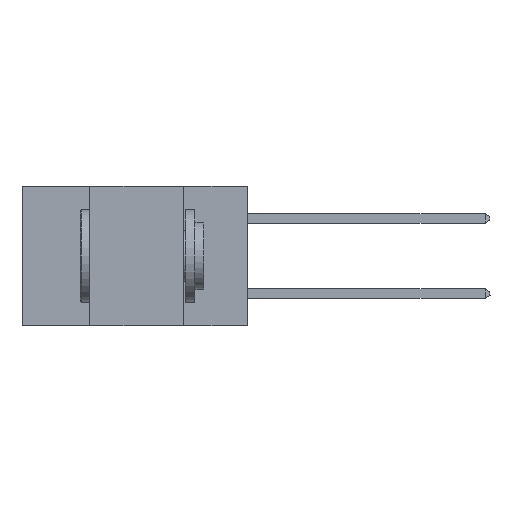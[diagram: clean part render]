
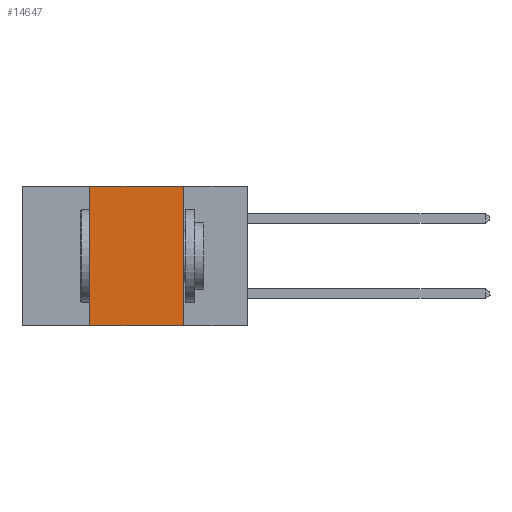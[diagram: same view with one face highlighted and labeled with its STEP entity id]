
A CAD part, left-side view. The second image highlights one B-rep face of the part: STEP entity #14647.
In plain terms, the highlighted planar face has unit normal (-1, 0, 0).
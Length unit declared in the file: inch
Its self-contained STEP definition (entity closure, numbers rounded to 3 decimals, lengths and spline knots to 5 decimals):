
#562 = PLANE ( 'NONE',  #14080 ) ;
#1736 = CARTESIAN_POINT ( 'NONE',  ( 0., 0.17, 0. ) ) ;
#3290 = VECTOR ( 'NONE', #17499, 39.37008 ) ;
#3989 = ORIENTED_EDGE ( 'NONE', *, *, #22649, .F. ) ;
#4442 = VERTEX_POINT ( 'NONE', #15856 ) ;
#6640 = CARTESIAN_POINT ( 'NONE',  ( 0., 0.6, 0. ) ) ;
#7183 = VECTOR ( 'NONE', #24436, 39.37008 ) ;
#7204 = ORIENTED_EDGE ( 'NONE', *, *, #22754, .T. ) ;
#7404 = LINE ( 'NONE', #11483, #8375 ) ;
#7886 = ORIENTED_EDGE ( 'NONE', *, *, #10504, .F. ) ;
#8375 = VECTOR ( 'NONE', #13555, 39.37008 ) ;
#9929 = VERTEX_POINT ( 'NONE', #11337 ) ;
#10027 = LINE ( 'NONE', #10076, #7183 ) ;
#10076 = CARTESIAN_POINT ( 'NONE',  ( 0., 0.42, 0. ) ) ;
#10504 = EDGE_CURVE ( 'NONE', #4442, #9929, #18807, .T. ) ;
#11337 = CARTESIAN_POINT ( 'NONE',  ( 0., 0.17, -0.37 ) ) ;
#11483 = CARTESIAN_POINT ( 'NONE',  ( 0., 0.6, 0. ) ) ;
#11975 = EDGE_LOOP ( 'NONE', ( #7886, #3989, #15514, #7204 ) ) ;
#13225 = FACE_OUTER_BOUND ( 'NONE', #11975, .T. ) ;
#13555 = DIRECTION ( 'NONE',  ( 0., -1., 0. ) ) ;
#13827 = CARTESIAN_POINT ( 'NONE',  ( 0., 0.6, -0.37 ) ) ;
#14080 = AXIS2_PLACEMENT_3D ( 'NONE', #6640, #22886, #24940 ) ;
#14647 = ADVANCED_FACE ( 'NONE', ( #13225 ), #562, .F. ) ;
#14692 = CARTESIAN_POINT ( 'NONE',  ( 0., 0.42, -0.37 ) ) ;
#15514 = ORIENTED_EDGE ( 'NONE', *, *, #16528, .F. ) ;
#15603 = VECTOR ( 'NONE', #16011, 39.37008 ) ;
#15856 = CARTESIAN_POINT ( 'NONE',  ( 0., 0.17, 0. ) ) ;
#16011 = DIRECTION ( 'NONE',  ( 0., -1., 0. ) ) ;
#16528 = EDGE_CURVE ( 'NONE', #24000, #17291, #10027, .T. ) ;
#17291 = VERTEX_POINT ( 'NONE', #20662 ) ;
#17499 = DIRECTION ( 'NONE',  ( 0., 0., -1. ) ) ;
#18807 = LINE ( 'NONE', #1736, #3290 ) ;
#20662 = CARTESIAN_POINT ( 'NONE',  ( 0., 0.42, 0. ) ) ;
#21060 = LINE ( 'NONE', #13827, #15603 ) ;
#22649 = EDGE_CURVE ( 'NONE', #17291, #4442, #7404, .T. ) ;
#22754 = EDGE_CURVE ( 'NONE', #24000, #9929, #21060, .T. ) ;
#22886 = DIRECTION ( 'NONE',  ( 1., 0., 0. ) ) ;
#24000 = VERTEX_POINT ( 'NONE', #14692 ) ;
#24436 = DIRECTION ( 'NONE',  ( 0., 0., 1. ) ) ;
#24940 = DIRECTION ( 'NONE',  ( 0., 0., -1. ) ) ;
